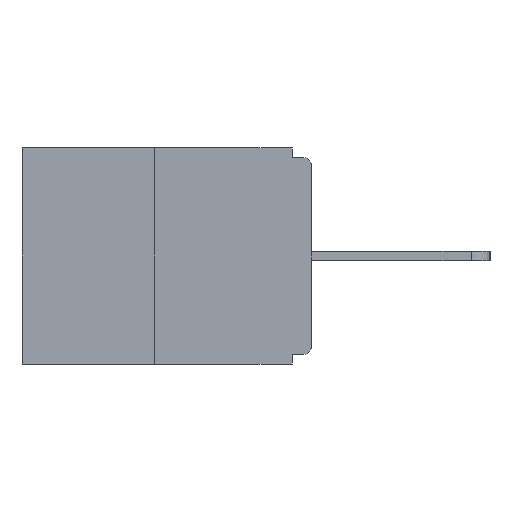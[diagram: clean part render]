
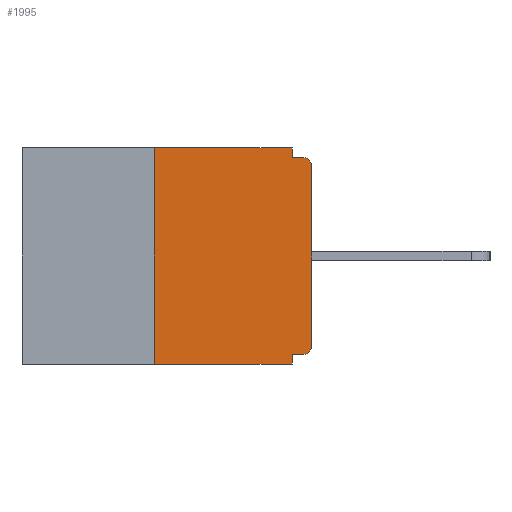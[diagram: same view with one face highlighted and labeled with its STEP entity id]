
A CAD part, left-side view. The second image highlights one B-rep face of the part: STEP entity #1995.
In plain terms, the highlighted planar face has unit normal (-1, 0, 0).
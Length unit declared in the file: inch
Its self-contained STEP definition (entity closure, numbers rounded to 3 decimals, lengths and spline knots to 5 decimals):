
#180 = EDGE_CURVE ( 'NONE', #15653, #9840, #2602, .T. ) ;
#990 = VECTOR ( 'NONE', #10599, 39.37008 ) ;
#1143 = ORIENTED_EDGE ( 'NONE', *, *, #14106, .T. ) ;
#1556 = LINE ( 'NONE', #11220, #15224 ) ;
#1568 = VERTEX_POINT ( 'NONE', #14979 ) ;
#1589 = CARTESIAN_POINT ( 'NONE',  ( 0., 0.015, -0.015 ) ) ;
#1601 = ORIENTED_EDGE ( 'NONE', *, *, #16848, .F. ) ;
#1768 = EDGE_CURVE ( 'NONE', #9840, #6317, #7101, .T. ) ;
#1801 = DIRECTION ( 'NONE',  ( 0., 0., -1. ) ) ;
#1981 = LINE ( 'NONE', #5837, #4925 ) ;
#1995 = ADVANCED_FACE ( 'NONE', ( #7085 ), #11168, .F. ) ;
#2060 = VECTOR ( 'NONE', #15508, 39.37008 ) ;
#2472 = EDGE_CURVE ( 'NONE', #6317, #9132, #1981, .T. ) ;
#2517 = CARTESIAN_POINT ( 'NONE',  ( 0., 0.25, 0. ) ) ;
#2602 = LINE ( 'NONE', #2517, #8708 ) ;
#2823 = DIRECTION ( 'NONE',  ( 1., 0., 0. ) ) ;
#3047 = CARTESIAN_POINT ( 'NONE',  ( 0., 0.25, -0.343 ) ) ;
#3061 = ORIENTED_EDGE ( 'NONE', *, *, #180, .F. ) ;
#3137 = DIRECTION ( 'NONE',  ( 0., 0., -1. ) ) ;
#4149 = AXIS2_PLACEMENT_3D ( 'NONE', #5788, #2823, #7170 ) ;
#4726 = VECTOR ( 'NONE', #13491, 39.37008 ) ;
#4811 = CARTESIAN_POINT ( 'NONE',  ( 0., 0.015, -0.03 ) ) ;
#4925 = VECTOR ( 'NONE', #1801, 39.37008 ) ;
#5078 = VECTOR ( 'NONE', #13799, 39.37008 ) ;
#5404 = EDGE_CURVE ( 'NONE', #15305, #7352, #9491, .T. ) ;
#5788 = CARTESIAN_POINT ( 'NONE',  ( 0., 0.46, 0. ) ) ;
#5837 = CARTESIAN_POINT ( 'NONE',  ( 0., 0.031, 0. ) ) ;
#6022 = EDGE_CURVE ( 'NONE', #1568, #15305, #6632, .T. ) ;
#6026 = DIRECTION ( 'NONE',  ( 0., 0., -1. ) ) ;
#6315 = ORIENTED_EDGE ( 'NONE', *, *, #6022, .T. ) ;
#6317 = VERTEX_POINT ( 'NONE', #8311 ) ;
#6533 = DIRECTION ( 'NONE',  ( 0., 0., 1. ) ) ;
#6562 = ORIENTED_EDGE ( 'NONE', *, *, #1768, .F. ) ;
#6628 = CARTESIAN_POINT ( 'NONE',  ( 0., 0., -0.015 ) ) ;
#6632 = CIRCLE ( 'NONE', #14688, 0.015 ) ;
#6808 = EDGE_LOOP ( 'NONE', ( #6562, #3061, #10108, #1601, #13290, #6315, #11437, #1143, #15140, #9417 ) ) ;
#7085 = FACE_OUTER_BOUND ( 'NONE', #6808, .T. ) ;
#7101 = LINE ( 'NONE', #16693, #5078 ) ;
#7170 = DIRECTION ( 'NONE',  ( 0., 0., -1. ) ) ;
#7352 = VERTEX_POINT ( 'NONE', #17120 ) ;
#7494 = CARTESIAN_POINT ( 'NONE',  ( 0., 0., -0.313 ) ) ;
#7522 = CARTESIAN_POINT ( 'NONE',  ( 0., 0.031, -0.343 ) ) ;
#7605 = CARTESIAN_POINT ( 'NONE',  ( 0., 0.031, -0.328 ) ) ;
#7631 = CARTESIAN_POINT ( 'NONE',  ( 0., 0.46, -0.343 ) ) ;
#7855 = VERTEX_POINT ( 'NONE', #7522 ) ;
#8311 = CARTESIAN_POINT ( 'NONE',  ( 0., 0.031, 0. ) ) ;
#8504 = VECTOR ( 'NONE', #14367, 39.37008 ) ;
#8708 = VECTOR ( 'NONE', #6533, 39.37008 ) ;
#9132 = VERTEX_POINT ( 'NONE', #11603 ) ;
#9193 = VERTEX_POINT ( 'NONE', #7605 ) ;
#9417 = ORIENTED_EDGE ( 'NONE', *, *, #2472, .F. ) ;
#9472 = CARTESIAN_POINT ( 'NONE',  ( 0., 0., -0.328 ) ) ;
#9491 = LINE ( 'NONE', #14892, #4726 ) ;
#9840 = VERTEX_POINT ( 'NONE', #12452 ) ;
#9931 = DIRECTION ( 'NONE',  ( -1., 0., 0. ) ) ;
#10108 = ORIENTED_EDGE ( 'NONE', *, *, #15811, .T. ) ;
#10599 = DIRECTION ( 'NONE',  ( 0., -1., 0. ) ) ;
#11168 = PLANE ( 'NONE',  #4149 ) ;
#11220 = CARTESIAN_POINT ( 'NONE',  ( 0., 0.031, -0.343 ) ) ;
#11368 = DIRECTION ( 'NONE',  ( -1., 0., 0. ) ) ;
#11437 = ORIENTED_EDGE ( 'NONE', *, *, #5404, .T. ) ;
#11603 = CARTESIAN_POINT ( 'NONE',  ( 0., 0.031, -0.015 ) ) ;
#11838 = CIRCLE ( 'NONE', #14075, 0.015 ) ;
#12009 = LINE ( 'NONE', #6628, #8504 ) ;
#12037 = EDGE_CURVE ( 'NONE', #1568, #9193, #17230, .T. ) ;
#12452 = CARTESIAN_POINT ( 'NONE',  ( 0., 0.25, 0. ) ) ;
#12935 = CARTESIAN_POINT ( 'NONE',  ( 0., 0.015, -0.313 ) ) ;
#13290 = ORIENTED_EDGE ( 'NONE', *, *, #12037, .F. ) ;
#13491 = DIRECTION ( 'NONE',  ( 0., 0., 1. ) ) ;
#13799 = DIRECTION ( 'NONE',  ( 0., -1., 0. ) ) ;
#14075 = AXIS2_PLACEMENT_3D ( 'NONE', #4811, #9931, #6026 ) ;
#14106 = EDGE_CURVE ( 'NONE', #7352, #14704, #11838, .T. ) ;
#14367 = DIRECTION ( 'NONE',  ( 0., -1., 0. ) ) ;
#14610 = LINE ( 'NONE', #7631, #990 ) ;
#14688 = AXIS2_PLACEMENT_3D ( 'NONE', #12935, #11368, #15642 ) ;
#14704 = VERTEX_POINT ( 'NONE', #1589 ) ;
#14892 = CARTESIAN_POINT ( 'NONE',  ( 0., 0., 0. ) ) ;
#14979 = CARTESIAN_POINT ( 'NONE',  ( 0., 0.015, -0.328 ) ) ;
#15140 = ORIENTED_EDGE ( 'NONE', *, *, #15397, .F. ) ;
#15224 = VECTOR ( 'NONE', #3137, 39.37008 ) ;
#15305 = VERTEX_POINT ( 'NONE', #7494 ) ;
#15397 = EDGE_CURVE ( 'NONE', #9132, #14704, #12009, .T. ) ;
#15508 = DIRECTION ( 'NONE',  ( 0., 1., 0. ) ) ;
#15642 = DIRECTION ( 'NONE',  ( 0., 0., -1. ) ) ;
#15653 = VERTEX_POINT ( 'NONE', #3047 ) ;
#15811 = EDGE_CURVE ( 'NONE', #15653, #7855, #14610, .T. ) ;
#16693 = CARTESIAN_POINT ( 'NONE',  ( 0., 0.46, 0. ) ) ;
#16848 = EDGE_CURVE ( 'NONE', #9193, #7855, #1556, .T. ) ;
#17120 = CARTESIAN_POINT ( 'NONE',  ( 0., 0., -0.03 ) ) ;
#17230 = LINE ( 'NONE', #9472, #2060 ) ;
